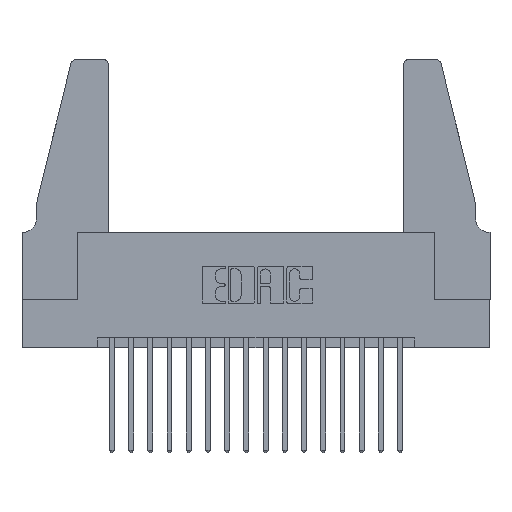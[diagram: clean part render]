
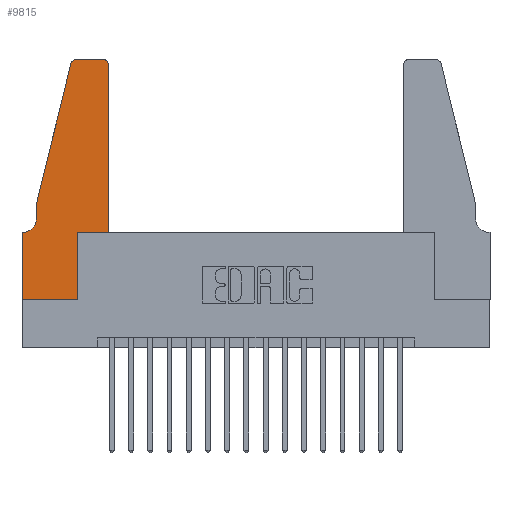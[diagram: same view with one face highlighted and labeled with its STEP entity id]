
A CAD part, top view. The second image highlights one B-rep face of the part: STEP entity #9815.
In plain terms, the highlighted planar face has unit normal (0, 0, 1).
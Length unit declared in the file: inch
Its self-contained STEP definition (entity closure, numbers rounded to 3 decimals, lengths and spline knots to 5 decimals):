
#125 = CARTESIAN_POINT ( 'NONE',  ( 0.284, 1.25, 0.37 ) ) ;
#278 = DIRECTION ( 'NONE',  ( 0., -1., 0. ) ) ;
#1067 = CARTESIAN_POINT ( 'NONE',  ( 0.0055, 0.42, 0.37 ) ) ;
#1272 = ORIENTED_EDGE ( 'NONE', *, *, #12048, .T. ) ;
#1328 = LINE ( 'NONE', #3759, #3094 ) ;
#1329 = VERTEX_POINT ( 'NONE', #125 ) ;
#1703 = AXIS2_PLACEMENT_3D ( 'NONE', #8958, #2364, #6987 ) ;
#1801 = VERTEX_POINT ( 'NONE', #9890 ) ;
#1881 = VECTOR ( 'NONE', #3810, 39.37008 ) ;
#2238 = LINE ( 'NONE', #4622, #3324 ) ;
#2364 = DIRECTION ( 'NONE',  ( 0., 0., 1. ) ) ;
#2731 = LINE ( 'NONE', #12060, #8913 ) ;
#2856 = DIRECTION ( 'NONE',  ( 0., 1., 0. ) ) ;
#2891 = ORIENTED_EDGE ( 'NONE', *, *, #10177, .T. ) ;
#3094 = VECTOR ( 'NONE', #8140, 39.37008 ) ;
#3235 = FACE_OUTER_BOUND ( 'NONE', #11273, .T. ) ;
#3324 = VECTOR ( 'NONE', #8710, 39.37008 ) ;
#3410 = ORIENTED_EDGE ( 'NONE', *, *, #12961, .T. ) ;
#3713 = ORIENTED_EDGE ( 'NONE', *, *, #16578, .T. ) ;
#3755 = LINE ( 'NONE', #14055, #18066 ) ;
#3759 = CARTESIAN_POINT ( 'NONE',  ( 0.0755, 0.5, 0.37 ) ) ;
#3810 = DIRECTION ( 'NONE',  ( 1., 0., 0. ) ) ;
#4305 = CARTESIAN_POINT ( 'NONE',  ( 0.25487, 1.22718, 0.37 ) ) ;
#4382 = CARTESIAN_POINT ( 'NONE',  ( 0., 0., 0.37 ) ) ;
#4622 = CARTESIAN_POINT ( 'NONE',  ( 0.0755, 0.5, 0.37 ) ) ;
#4695 = LINE ( 'NONE', #7002, #8671 ) ;
#4721 = ORIENTED_EDGE ( 'NONE', *, *, #10482, .T. ) ;
#5247 = ORIENTED_EDGE ( 'NONE', *, *, #12935, .T. ) ;
#5279 = ORIENTED_EDGE ( 'NONE', *, *, #7805, .T. ) ;
#5829 = VERTEX_POINT ( 'NONE', #16568 ) ;
#6338 = ORIENTED_EDGE ( 'NONE', *, *, #9290, .T. ) ;
#6435 = AXIS2_PLACEMENT_3D ( 'NONE', #13438, #8060, #17761 ) ;
#6546 = DIRECTION ( 'NONE',  ( 0., 0., -1. ) ) ;
#6641 = VERTEX_POINT ( 'NONE', #9486 ) ;
#6963 = CARTESIAN_POINT ( 'NONE',  ( 0.0755, 0.5, 0.37 ) ) ;
#6987 = DIRECTION ( 'NONE',  ( 1., 0., 0. ) ) ;
#7002 = CARTESIAN_POINT ( 'NONE',  ( 0.2865, 0.35, 0.37 ) ) ;
#7074 = DIRECTION ( 'NONE',  ( -1., 0., 0. ) ) ;
#7313 = EDGE_CURVE ( 'NONE', #8667, #16791, #4695, .T. ) ;
#7352 = DIRECTION ( 'NONE',  ( 0., 0., 1. ) ) ;
#7748 = LINE ( 'NONE', #4382, #9230 ) ;
#7805 = EDGE_CURVE ( 'NONE', #13443, #9639, #7748, .T. ) ;
#8060 = DIRECTION ( 'NONE',  ( 0., 0., 1. ) ) ;
#8077 = LINE ( 'NONE', #14382, #13986 ) ;
#8140 = DIRECTION ( 'NONE',  ( 0., -1., 0. ) ) ;
#8344 = CIRCLE ( 'NONE', #6435, 0.03 ) ;
#8451 = VECTOR ( 'NONE', #10428, 39.37008 ) ;
#8573 = VERTEX_POINT ( 'NONE', #4305 ) ;
#8600 = PLANE ( 'NONE',  #1703 ) ;
#8667 = VERTEX_POINT ( 'NONE', #16897 ) ;
#8671 = VECTOR ( 'NONE', #2856, 39.37008 ) ;
#8710 = DIRECTION ( 'NONE',  ( -0.239, -0.971, 0. ) ) ;
#8892 = CARTESIAN_POINT ( 'NONE',  ( 0., 0., 0.37 ) ) ;
#8896 = AXIS2_PLACEMENT_3D ( 'NONE', #11769, #7352, #17670 ) ;
#8913 = VECTOR ( 'NONE', #10682, 39.37008 ) ;
#8958 = CARTESIAN_POINT ( 'NONE',  ( 0., 0.35, 0.37 ) ) ;
#9145 = ORIENTED_EDGE ( 'NONE', *, *, #13360, .T. ) ;
#9230 = VECTOR ( 'NONE', #278, 39.37008 ) ;
#9277 = CIRCLE ( 'NONE', #8896, 0.03 ) ;
#9290 = EDGE_CURVE ( 'NONE', #1801, #5829, #8344, .T. ) ;
#9402 = VERTEX_POINT ( 'NONE', #10695 ) ;
#9486 = CARTESIAN_POINT ( 'NONE',  ( 0.0055, 0.35, 0.37 ) ) ;
#9639 = VERTEX_POINT ( 'NONE', #10142 ) ;
#9815 = ADVANCED_FACE ( 'NONE', ( #3235 ), #8600, .T. ) ;
#9890 = CARTESIAN_POINT ( 'NONE',  ( 0.4505, 1.22, 0.37 ) ) ;
#10142 = CARTESIAN_POINT ( 'NONE',  ( 0., 0., 0.37 ) ) ;
#10177 = EDGE_CURVE ( 'NONE', #6641, #13443, #8077, .T. ) ;
#10428 = DIRECTION ( 'NONE',  ( 1., 0., 0. ) ) ;
#10482 = EDGE_CURVE ( 'NONE', #16791, #16857, #17736, .T. ) ;
#10682 = DIRECTION ( 'NONE',  ( 0., 1., 0. ) ) ;
#10695 = CARTESIAN_POINT ( 'NONE',  ( 0.0755, 0.42, 0.37 ) ) ;
#10894 = EDGE_CURVE ( 'NONE', #16857, #1801, #2731, .T. ) ;
#11273 = EDGE_LOOP ( 'NONE', ( #9145, #3713, #5247, #14433, #3410, #2891, #5279, #1272, #16187, #4721, #11962, #6338 ) ) ;
#11769 = CARTESIAN_POINT ( 'NONE',  ( 0.284, 1.22, 0.37 ) ) ;
#11962 = ORIENTED_EDGE ( 'NONE', *, *, #10894, .T. ) ;
#12048 = EDGE_CURVE ( 'NONE', #9639, #8667, #12190, .T. ) ;
#12060 = CARTESIAN_POINT ( 'NONE',  ( 0.4505, 0.35, 0.37 ) ) ;
#12190 = LINE ( 'NONE', #8892, #8451 ) ;
#12935 = EDGE_CURVE ( 'NONE', #8573, #16774, #2238, .T. ) ;
#12961 = EDGE_CURVE ( 'NONE', #9402, #6641, #16101, .T. ) ;
#13360 = EDGE_CURVE ( 'NONE', #5829, #1329, #3755, .T. ) ;
#13384 = EDGE_CURVE ( 'NONE', #16774, #9402, #1328, .T. ) ;
#13438 = CARTESIAN_POINT ( 'NONE',  ( 0.4205, 1.22, 0.37 ) ) ;
#13443 = VERTEX_POINT ( 'NONE', #17727 ) ;
#13857 = AXIS2_PLACEMENT_3D ( 'NONE', #1067, #6546, #14915 ) ;
#13965 = CARTESIAN_POINT ( 'NONE',  ( 0.4505, 0.35, 0.37 ) ) ;
#13986 = VECTOR ( 'NONE', #7074, 39.37008 ) ;
#14007 = CARTESIAN_POINT ( 'NONE',  ( 0.2865, 0.35, 0.37 ) ) ;
#14055 = CARTESIAN_POINT ( 'NONE',  ( 0.2605, 1.25, 0.37 ) ) ;
#14382 = CARTESIAN_POINT ( 'NONE',  ( 0.0755, 0.35, 0.37 ) ) ;
#14433 = ORIENTED_EDGE ( 'NONE', *, *, #13384, .T. ) ;
#14915 = DIRECTION ( 'NONE',  ( -1., 0., 0. ) ) ;
#16101 = CIRCLE ( 'NONE', #13857, 0.07 ) ;
#16187 = ORIENTED_EDGE ( 'NONE', *, *, #7313, .T. ) ;
#16568 = CARTESIAN_POINT ( 'NONE',  ( 0.4205, 1.25, 0.37 ) ) ;
#16578 = EDGE_CURVE ( 'NONE', #1329, #8573, #9277, .T. ) ;
#16674 = CARTESIAN_POINT ( 'NONE',  ( 0.4505, 0.35, 0.37 ) ) ;
#16774 = VERTEX_POINT ( 'NONE', #6963 ) ;
#16791 = VERTEX_POINT ( 'NONE', #14007 ) ;
#16857 = VERTEX_POINT ( 'NONE', #13965 ) ;
#16897 = CARTESIAN_POINT ( 'NONE',  ( 0.2865, 0., 0.37 ) ) ;
#17451 = DIRECTION ( 'NONE',  ( -1., 0., 0. ) ) ;
#17670 = DIRECTION ( 'NONE',  ( 1., 0., 0. ) ) ;
#17727 = CARTESIAN_POINT ( 'NONE',  ( 0., 0.35, 0.37 ) ) ;
#17736 = LINE ( 'NONE', #16674, #1881 ) ;
#17761 = DIRECTION ( 'NONE',  ( 1., 0., 0. ) ) ;
#18066 = VECTOR ( 'NONE', #17451, 39.37008 ) ;
